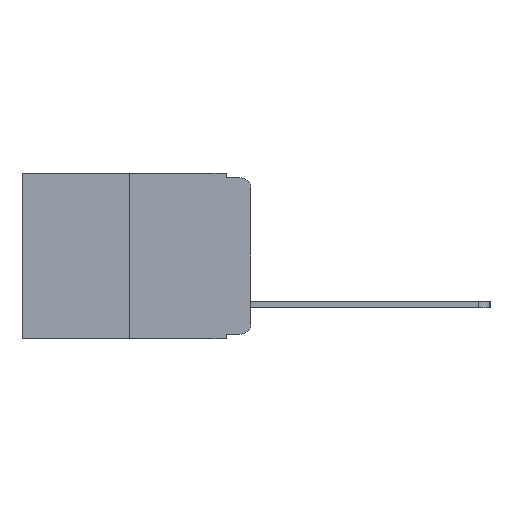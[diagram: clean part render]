
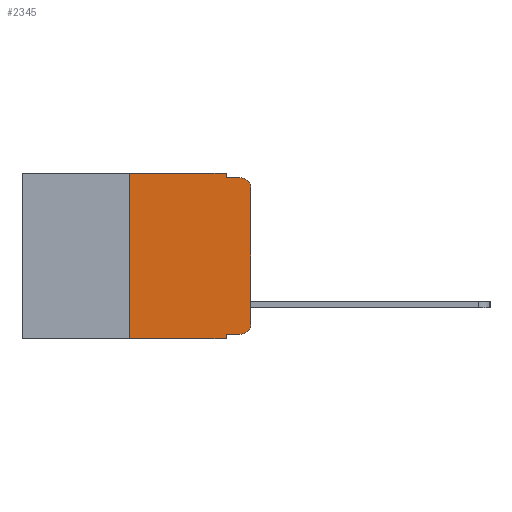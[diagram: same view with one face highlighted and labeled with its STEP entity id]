
A CAD part, left-side view. The second image highlights one B-rep face of the part: STEP entity #2345.
In plain terms, the highlighted planar face has unit normal (-1, 0, 0).
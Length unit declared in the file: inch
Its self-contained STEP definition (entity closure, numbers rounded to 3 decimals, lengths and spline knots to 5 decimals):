
#299 = LINE ( 'NONE', #9236, #2561 ) ;
#311 = CARTESIAN_POINT ( 'NONE',  ( 0., 0.02, -0.313 ) ) ;
#547 = AXIS2_PLACEMENT_3D ( 'NONE', #9816, #9900, #10912 ) ;
#765 = ORIENTED_EDGE ( 'NONE', *, *, #7028, .T. ) ;
#939 = LINE ( 'NONE', #7336, #10790 ) ;
#997 = CARTESIAN_POINT ( 'NONE',  ( 0., 0.25, 0. ) ) ;
#1344 = CARTESIAN_POINT ( 'NONE',  ( 0., 0.02, -0.333 ) ) ;
#1385 = EDGE_LOOP ( 'NONE', ( #2861, #765, #8150, #9278, #7638, #6890, #8955, #9673, #7310, #11597 ) ) ;
#1409 = DIRECTION ( 'NONE',  ( 0., 0., -1. ) ) ;
#1854 = VERTEX_POINT ( 'NONE', #2720 ) ;
#2327 = CARTESIAN_POINT ( 'NONE',  ( 0., 0.02, -0.01 ) ) ;
#2345 = ADVANCED_FACE ( 'NONE', ( #7341 ), #9839, .F. ) ;
#2349 = VERTEX_POINT ( 'NONE', #10882 ) ;
#2379 = EDGE_CURVE ( 'NONE', #8821, #10653, #939, .T. ) ;
#2450 = AXIS2_PLACEMENT_3D ( 'NONE', #10675, #5659, #11429 ) ;
#2561 = VECTOR ( 'NONE', #10027, 39.37008 ) ;
#2720 = CARTESIAN_POINT ( 'NONE',  ( 0., 0.051, -0.333 ) ) ;
#2861 = ORIENTED_EDGE ( 'NONE', *, *, #6982, .T. ) ;
#3216 = VERTEX_POINT ( 'NONE', #2327 ) ;
#3323 = CARTESIAN_POINT ( 'NONE',  ( 0., 0., 0. ) ) ;
#3337 = LINE ( 'NONE', #7543, #10604 ) ;
#3637 = CARTESIAN_POINT ( 'NONE',  ( 0., 0.25, 0. ) ) ;
#3739 = VECTOR ( 'NONE', #10445, 39.37008 ) ;
#4067 = VECTOR ( 'NONE', #10607, 39.37008 ) ;
#4218 = LINE ( 'NONE', #4843, #9168 ) ;
#4571 = CIRCLE ( 'NONE', #11112, 0.02 ) ;
#4843 = CARTESIAN_POINT ( 'NONE',  ( 0., 0.051, -0.333 ) ) ;
#4924 = VECTOR ( 'NONE', #10797, 39.37008 ) ;
#5613 = LINE ( 'NONE', #11516, #4924 ) ;
#5659 = DIRECTION ( 'NONE',  ( -1., 0., 0. ) ) ;
#6004 = CARTESIAN_POINT ( 'NONE',  ( 0., 0.051, 0. ) ) ;
#6024 = EDGE_CURVE ( 'NONE', #2349, #7248, #8584, .T. ) ;
#6138 = VERTEX_POINT ( 'NONE', #7390 ) ;
#6535 = CIRCLE ( 'NONE', #2450, 0.02 ) ;
#6890 = ORIENTED_EDGE ( 'NONE', *, *, #7126, .F. ) ;
#6982 = EDGE_CURVE ( 'NONE', #8947, #6138, #11070, .T. ) ;
#7028 = EDGE_CURVE ( 'NONE', #6138, #3216, #6535, .T. ) ;
#7069 = EDGE_CURVE ( 'NONE', #9412, #3216, #3337, .T. ) ;
#7111 = EDGE_CURVE ( 'NONE', #10653, #9412, #299, .T. ) ;
#7126 = EDGE_CURVE ( 'NONE', #2349, #8821, #9661, .T. ) ;
#7128 = EDGE_CURVE ( 'NONE', #1854, #7248, #5613, .T. ) ;
#7146 = EDGE_CURVE ( 'NONE', #1854, #10387, #4218, .T. ) ;
#7151 = EDGE_CURVE ( 'NONE', #10387, #8947, #4571, .T. ) ;
#7248 = VERTEX_POINT ( 'NONE', #7893 ) ;
#7310 = ORIENTED_EDGE ( 'NONE', *, *, #7146, .T. ) ;
#7336 = CARTESIAN_POINT ( 'NONE',  ( 0., 0.473, 0. ) ) ;
#7341 = FACE_OUTER_BOUND ( 'NONE', #1385, .T. ) ;
#7390 = CARTESIAN_POINT ( 'NONE',  ( 0., 0., -0.03 ) ) ;
#7409 = DIRECTION ( 'NONE',  ( 0., -1., 0. ) ) ;
#7543 = CARTESIAN_POINT ( 'NONE',  ( 0., 0.051, -0.01 ) ) ;
#7638 = ORIENTED_EDGE ( 'NONE', *, *, #2379, .F. ) ;
#7778 = DIRECTION ( 'NONE',  ( -1., 0., 0. ) ) ;
#7893 = CARTESIAN_POINT ( 'NONE',  ( 0., 0.051, -0.343 ) ) ;
#8150 = ORIENTED_EDGE ( 'NONE', *, *, #7069, .F. ) ;
#8584 = LINE ( 'NONE', #8921, #3739 ) ;
#8821 = VERTEX_POINT ( 'NONE', #997 ) ;
#8921 = CARTESIAN_POINT ( 'NONE',  ( 0., 0.473, -0.343 ) ) ;
#8947 = VERTEX_POINT ( 'NONE', #9167 ) ;
#8955 = ORIENTED_EDGE ( 'NONE', *, *, #6024, .T. ) ;
#9167 = CARTESIAN_POINT ( 'NONE',  ( 0., 0., -0.313 ) ) ;
#9168 = VECTOR ( 'NONE', #10865, 39.37008 ) ;
#9236 = CARTESIAN_POINT ( 'NONE',  ( 0., 0.051, 0. ) ) ;
#9278 = ORIENTED_EDGE ( 'NONE', *, *, #7111, .F. ) ;
#9412 = VERTEX_POINT ( 'NONE', #10189 ) ;
#9661 = LINE ( 'NONE', #3637, #11665 ) ;
#9673 = ORIENTED_EDGE ( 'NONE', *, *, #7128, .F. ) ;
#9816 = CARTESIAN_POINT ( 'NONE',  ( 0., 0.473, 0. ) ) ;
#9839 = PLANE ( 'NONE',  #547 ) ;
#9900 = DIRECTION ( 'NONE',  ( 1., 0., 0. ) ) ;
#9963 = DIRECTION ( 'NONE',  ( 0., -1., 0. ) ) ;
#10027 = DIRECTION ( 'NONE',  ( 0., 0., -1. ) ) ;
#10064 = DIRECTION ( 'NONE',  ( 0., 0., 1. ) ) ;
#10189 = CARTESIAN_POINT ( 'NONE',  ( 0., 0.051, -0.01 ) ) ;
#10387 = VERTEX_POINT ( 'NONE', #1344 ) ;
#10445 = DIRECTION ( 'NONE',  ( 0., -1., 0. ) ) ;
#10604 = VECTOR ( 'NONE', #9963, 39.37008 ) ;
#10607 = DIRECTION ( 'NONE',  ( 0., 0., 1. ) ) ;
#10653 = VERTEX_POINT ( 'NONE', #6004 ) ;
#10675 = CARTESIAN_POINT ( 'NONE',  ( 0., 0.02, -0.03 ) ) ;
#10790 = VECTOR ( 'NONE', #7409, 39.37008 ) ;
#10797 = DIRECTION ( 'NONE',  ( 0., 0., -1. ) ) ;
#10865 = DIRECTION ( 'NONE',  ( 0., -1., 0. ) ) ;
#10882 = CARTESIAN_POINT ( 'NONE',  ( 0., 0.25, -0.343 ) ) ;
#10912 = DIRECTION ( 'NONE',  ( 0., 0., -1. ) ) ;
#11070 = LINE ( 'NONE', #3323, #4067 ) ;
#11112 = AXIS2_PLACEMENT_3D ( 'NONE', #311, #7778, #1409 ) ;
#11429 = DIRECTION ( 'NONE',  ( 0., 0., -1. ) ) ;
#11516 = CARTESIAN_POINT ( 'NONE',  ( 0., 0.051, 0. ) ) ;
#11597 = ORIENTED_EDGE ( 'NONE', *, *, #7151, .T. ) ;
#11665 = VECTOR ( 'NONE', #10064, 39.37008 ) ;
